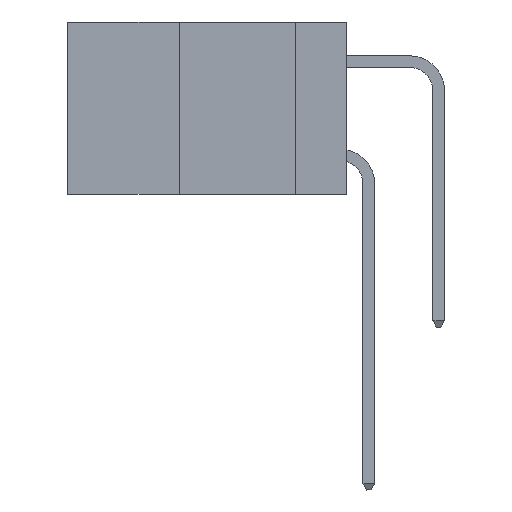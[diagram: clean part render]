
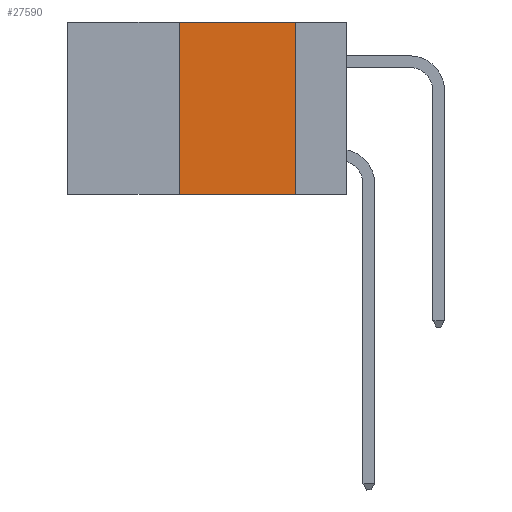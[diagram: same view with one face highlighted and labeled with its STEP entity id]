
A CAD part, left-side view. The second image highlights one B-rep face of the part: STEP entity #27590.
In plain terms, the highlighted planar face has unit normal (-1, 0, 0).
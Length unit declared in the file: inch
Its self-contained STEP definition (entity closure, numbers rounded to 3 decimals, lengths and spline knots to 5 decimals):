
#33 = AXIS2_PLACEMENT_3D ( 'NONE', #8844, #4154, #24809 ) ;
#73 = VERTEX_POINT ( 'NONE', #12851 ) ;
#612 = CARTESIAN_POINT ( 'NONE',  ( 0., 0.6, -0.37 ) ) ;
#2336 = EDGE_LOOP ( 'NONE', ( #13896, #22580, #12189, #23091 ) ) ;
#3537 = DIRECTION ( 'NONE',  ( 0., -1., 0. ) ) ;
#3639 = CARTESIAN_POINT ( 'NONE',  ( 0., 0.6, 0. ) ) ;
#3903 = VECTOR ( 'NONE', #17298, 39.37008 ) ;
#4154 = DIRECTION ( 'NONE',  ( 1., 0., 0. ) ) ;
#4515 = DIRECTION ( 'NONE',  ( 0., 0., 1. ) ) ;
#5613 = CARTESIAN_POINT ( 'NONE',  ( 0., 0.11, 0. ) ) ;
#5621 = VERTEX_POINT ( 'NONE', #6476 ) ;
#6476 = CARTESIAN_POINT ( 'NONE',  ( 0., 0.11, -0.37 ) ) ;
#8561 = VERTEX_POINT ( 'NONE', #22436 ) ;
#8844 = CARTESIAN_POINT ( 'NONE',  ( 0., 0.6, 0. ) ) ;
#9074 = LINE ( 'NONE', #22504, #24416 ) ;
#10470 = EDGE_CURVE ( 'NONE', #73, #24769, #9074, .T. ) ;
#11771 = LINE ( 'NONE', #612, #15677 ) ;
#12189 = ORIENTED_EDGE ( 'NONE', *, *, #10470, .F. ) ;
#12524 = LINE ( 'NONE', #3639, #24292 ) ;
#12554 = EDGE_CURVE ( 'NONE', #8561, #5621, #18561, .T. ) ;
#12851 = CARTESIAN_POINT ( 'NONE',  ( 0., 0.36, -0.37 ) ) ;
#13896 = ORIENTED_EDGE ( 'NONE', *, *, #12554, .F. ) ;
#14280 = FACE_OUTER_BOUND ( 'NONE', #2336, .T. ) ;
#14350 = DIRECTION ( 'NONE',  ( 0., -1., 0. ) ) ;
#15677 = VECTOR ( 'NONE', #14350, 39.37008 ) ;
#17298 = DIRECTION ( 'NONE',  ( 0., 0., -1. ) ) ;
#18561 = LINE ( 'NONE', #5613, #3903 ) ;
#19060 = EDGE_CURVE ( 'NONE', #24769, #8561, #12524, .T. ) ;
#19560 = CARTESIAN_POINT ( 'NONE',  ( 0., 0.36, 0. ) ) ;
#22436 = CARTESIAN_POINT ( 'NONE',  ( 0., 0.11, 0. ) ) ;
#22504 = CARTESIAN_POINT ( 'NONE',  ( 0., 0.36, 0. ) ) ;
#22580 = ORIENTED_EDGE ( 'NONE', *, *, #19060, .F. ) ;
#22780 = EDGE_CURVE ( 'NONE', #73, #5621, #11771, .T. ) ;
#23091 = ORIENTED_EDGE ( 'NONE', *, *, #22780, .T. ) ;
#24292 = VECTOR ( 'NONE', #3537, 39.37008 ) ;
#24416 = VECTOR ( 'NONE', #4515, 39.37008 ) ;
#24769 = VERTEX_POINT ( 'NONE', #19560 ) ;
#24809 = DIRECTION ( 'NONE',  ( 0., 0., -1. ) ) ;
#26666 = PLANE ( 'NONE',  #33 ) ;
#27590 = ADVANCED_FACE ( 'NONE', ( #14280 ), #26666, .F. ) ;
